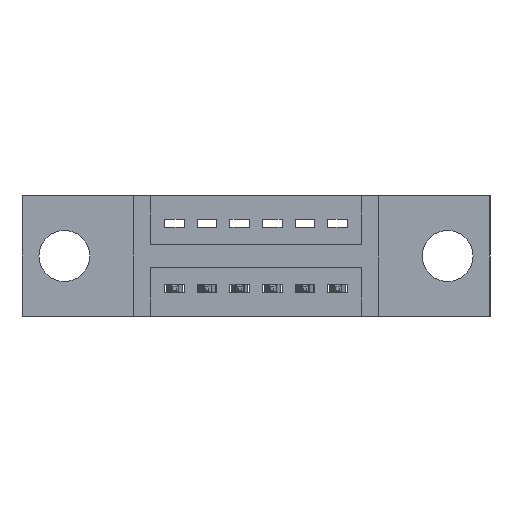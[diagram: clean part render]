
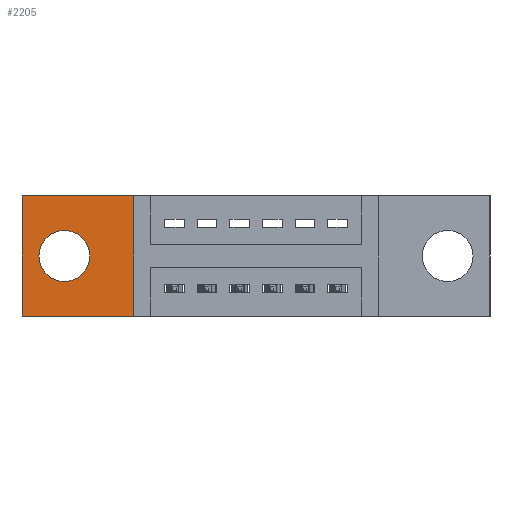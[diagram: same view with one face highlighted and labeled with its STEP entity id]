
A CAD part, front view. The second image highlights one B-rep face of the part: STEP entity #2205.
In plain terms, the highlighted planar face has unit normal (0, -1, 0).
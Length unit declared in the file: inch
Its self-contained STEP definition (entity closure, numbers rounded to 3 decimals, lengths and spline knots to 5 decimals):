
#11 = DIRECTION ( 'NONE',  ( 0., -1., 0. ) ) ;
#71 = ORIENTED_EDGE ( 'NONE', *, *, #8959, .F. ) ;
#85 = ORIENTED_EDGE ( 'NONE', *, *, #641, .F. ) ;
#146 = ORIENTED_EDGE ( 'NONE', *, *, #3193, .T. ) ;
#218 = ORIENTED_EDGE ( 'NONE', *, *, #8796, .T. ) ;
#260 = ORIENTED_EDGE ( 'NONE', *, *, #9070, .T. ) ;
#502 = ORIENTED_EDGE ( 'NONE', *, *, #2239, .T. ) ;
#641 = EDGE_CURVE ( 'NONE', #4804, #4750, #6170, .T. ) ;
#1098 = VERTEX_POINT ( 'NONE', #6742 ) ;
#1312 = CARTESIAN_POINT ( 'NONE',  ( 0.3425, 0.17, 0. ) ) ;
#1961 = CARTESIAN_POINT ( 'NONE',  ( 0.3425, 0.17, 0. ) ) ;
#2064 = DIRECTION ( 'NONE',  ( 0., -1., 0. ) ) ;
#2114 = CARTESIAN_POINT ( 'NONE',  ( 0.13, 0.17, -0.263 ) ) ;
#2205 = ADVANCED_FACE ( 'NONE', ( #7933, #6137 ), #2935, .T. ) ;
#2218 = CIRCLE ( 'NONE', #6681, 0.078 ) ;
#2239 = EDGE_CURVE ( 'NONE', #3356, #1098, #7753, .T. ) ;
#2334 = DIRECTION ( 'NONE',  ( -1., 0., 0. ) ) ;
#2374 = CARTESIAN_POINT ( 'NONE',  ( 0., 0.17, 0. ) ) ;
#2840 = DIRECTION ( 'NONE',  ( 0., 0., -1. ) ) ;
#2887 = DIRECTION ( 'NONE',  ( 0., -1., 0. ) ) ;
#2935 = PLANE ( 'NONE',  #5326 ) ;
#3193 = EDGE_CURVE ( 'NONE', #1098, #4860, #3510, .T. ) ;
#3356 = VERTEX_POINT ( 'NONE', #1961 ) ;
#3401 = CARTESIAN_POINT ( 'NONE',  ( 0., 0.17, -0.37 ) ) ;
#3510 = LINE ( 'NONE', #5299, #7011 ) ;
#3870 = CARTESIAN_POINT ( 'NONE',  ( 0.13, 0.17, -0.107 ) ) ;
#4173 = LINE ( 'NONE', #8420, #8182 ) ;
#4188 = DIRECTION ( 'NONE',  ( 1., 0., 0. ) ) ;
#4273 = EDGE_LOOP ( 'NONE', ( #146, #218, #260, #502 ) ) ;
#4404 = VERTEX_POINT ( 'NONE', #8225 ) ;
#4750 = VERTEX_POINT ( 'NONE', #3870 ) ;
#4804 = VERTEX_POINT ( 'NONE', #2114 ) ;
#4860 = VERTEX_POINT ( 'NONE', #8157 ) ;
#4908 = VECTOR ( 'NONE', #9229, 39.37008 ) ;
#5033 = EDGE_LOOP ( 'NONE', ( #71, #85 ) ) ;
#5185 = DIRECTION ( 'NONE',  ( 0., 0., -1. ) ) ;
#5299 = CARTESIAN_POINT ( 'NONE',  ( 0., 0.17, 0. ) ) ;
#5326 = AXIS2_PLACEMENT_3D ( 'NONE', #3401, #2887, #2840 ) ;
#5882 = VECTOR ( 'NONE', #2334, 39.37008 ) ;
#6137 = FACE_OUTER_BOUND ( 'NONE', #4273, .T. ) ;
#6170 = CIRCLE ( 'NONE', #6257, 0.078 ) ;
#6257 = AXIS2_PLACEMENT_3D ( 'NONE', #9533, #11, #7701 ) ;
#6652 = CARTESIAN_POINT ( 'NONE',  ( 0.13, 0.17, -0.185 ) ) ;
#6681 = AXIS2_PLACEMENT_3D ( 'NONE', #6652, #2064, #7326 ) ;
#6742 = CARTESIAN_POINT ( 'NONE',  ( 0., 0.17, 0. ) ) ;
#6848 = LINE ( 'NONE', #1312, #4908 ) ;
#7011 = VECTOR ( 'NONE', #5185, 39.37008 ) ;
#7326 = DIRECTION ( 'NONE',  ( 0., 0., -1. ) ) ;
#7701 = DIRECTION ( 'NONE',  ( 0., 0., -1. ) ) ;
#7753 = LINE ( 'NONE', #2374, #5882 ) ;
#7933 = FACE_BOUND ( 'NONE', #5033, .T. ) ;
#8157 = CARTESIAN_POINT ( 'NONE',  ( 0., 0.17, -0.37 ) ) ;
#8182 = VECTOR ( 'NONE', #4188, 39.37008 ) ;
#8225 = CARTESIAN_POINT ( 'NONE',  ( 0.3425, 0.17, -0.37 ) ) ;
#8420 = CARTESIAN_POINT ( 'NONE',  ( 0., 0.17, -0.37 ) ) ;
#8796 = EDGE_CURVE ( 'NONE', #4860, #4404, #4173, .T. ) ;
#8959 = EDGE_CURVE ( 'NONE', #4750, #4804, #2218, .T. ) ;
#9070 = EDGE_CURVE ( 'NONE', #4404, #3356, #6848, .T. ) ;
#9229 = DIRECTION ( 'NONE',  ( 0., 0., 1. ) ) ;
#9533 = CARTESIAN_POINT ( 'NONE',  ( 0.13, 0.17, -0.185 ) ) ;
